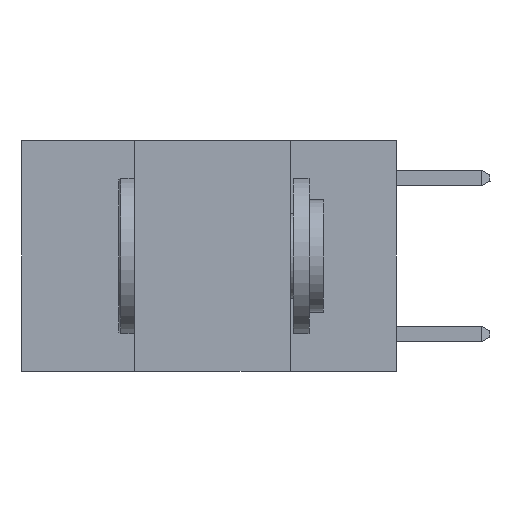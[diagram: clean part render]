
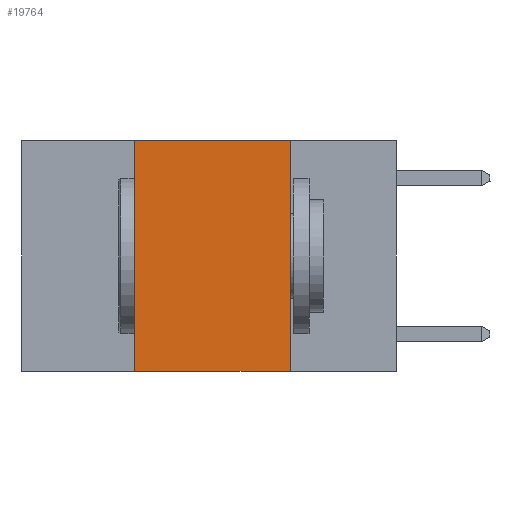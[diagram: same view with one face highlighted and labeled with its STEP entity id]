
A CAD part, left-side view. The second image highlights one B-rep face of the part: STEP entity #19764.
In plain terms, the highlighted planar face has unit normal (-1, 0, 0).
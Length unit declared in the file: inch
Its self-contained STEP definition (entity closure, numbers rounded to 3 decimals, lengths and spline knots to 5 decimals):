
#243 = VERTEX_POINT ( 'NONE', #7883 ) ;
#1084 = VECTOR ( 'NONE', #1887, 39.37008 ) ;
#1754 = CARTESIAN_POINT ( 'NONE',  ( 0., 0.17, -0.37 ) ) ;
#1887 = DIRECTION ( 'NONE',  ( 0., 0., 1. ) ) ;
#4046 = AXIS2_PLACEMENT_3D ( 'NONE', #18492, #10066, #21758 ) ;
#4828 = ORIENTED_EDGE ( 'NONE', *, *, #21207, .F. ) ;
#5165 = VECTOR ( 'NONE', #5549, 39.37008 ) ;
#5549 = DIRECTION ( 'NONE',  ( 0., -1., 0. ) ) ;
#6060 = CARTESIAN_POINT ( 'NONE',  ( 0., 0.17, 0. ) ) ;
#6267 = LINE ( 'NONE', #10755, #5165 ) ;
#7650 = VECTOR ( 'NONE', #7688, 39.37008 ) ;
#7688 = DIRECTION ( 'NONE',  ( 0., -1., 0. ) ) ;
#7883 = CARTESIAN_POINT ( 'NONE',  ( 0., 0.42, 0. ) ) ;
#8359 = PLANE ( 'NONE',  #4046 ) ;
#10066 = DIRECTION ( 'NONE',  ( 1., 0., 0. ) ) ;
#10597 = EDGE_LOOP ( 'NONE', ( #4828, #11100, #11203, #11283 ) ) ;
#10755 = CARTESIAN_POINT ( 'NONE',  ( 0., 0.6, -0.37 ) ) ;
#11100 = ORIENTED_EDGE ( 'NONE', *, *, #17601, .F. ) ;
#11152 = EDGE_CURVE ( 'NONE', #18079, #17315, #6267, .T. ) ;
#11203 = ORIENTED_EDGE ( 'NONE', *, *, #17921, .F. ) ;
#11283 = ORIENTED_EDGE ( 'NONE', *, *, #11152, .T. ) ;
#12896 = CARTESIAN_POINT ( 'NONE',  ( 0., 0.17, 0. ) ) ;
#14475 = CARTESIAN_POINT ( 'NONE',  ( 0., 0.6, 0. ) ) ;
#14829 = LINE ( 'NONE', #20571, #1084 ) ;
#15546 = VECTOR ( 'NONE', #19609, 39.37008 ) ;
#16662 = LINE ( 'NONE', #14475, #7650 ) ;
#16970 = VERTEX_POINT ( 'NONE', #12896 ) ;
#17315 = VERTEX_POINT ( 'NONE', #1754 ) ;
#17601 = EDGE_CURVE ( 'NONE', #243, #16970, #16662, .T. ) ;
#17921 = EDGE_CURVE ( 'NONE', #18079, #243, #14829, .T. ) ;
#18079 = VERTEX_POINT ( 'NONE', #19347 ) ;
#18157 = FACE_OUTER_BOUND ( 'NONE', #10597, .T. ) ;
#18492 = CARTESIAN_POINT ( 'NONE',  ( 0., 0.6, 0. ) ) ;
#19347 = CARTESIAN_POINT ( 'NONE',  ( 0., 0.42, -0.37 ) ) ;
#19609 = DIRECTION ( 'NONE',  ( 0., 0., -1. ) ) ;
#19764 = ADVANCED_FACE ( 'NONE', ( #18157 ), #8359, .F. ) ;
#19960 = LINE ( 'NONE', #6060, #15546 ) ;
#20571 = CARTESIAN_POINT ( 'NONE',  ( 0., 0.42, 0. ) ) ;
#21207 = EDGE_CURVE ( 'NONE', #16970, #17315, #19960, .T. ) ;
#21758 = DIRECTION ( 'NONE',  ( 0., 0., -1. ) ) ;
